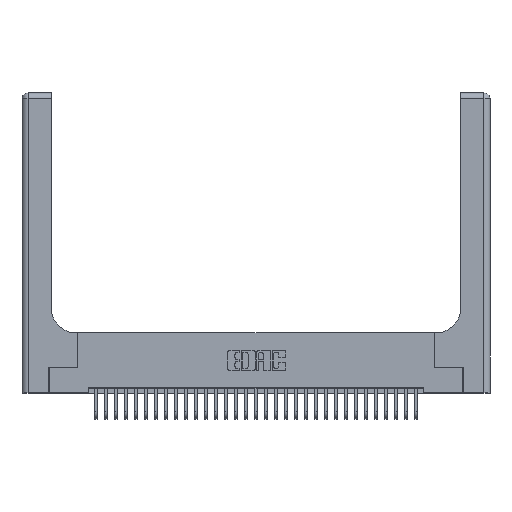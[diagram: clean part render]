
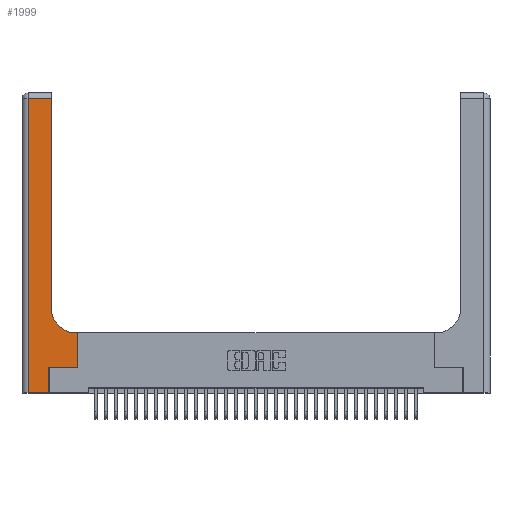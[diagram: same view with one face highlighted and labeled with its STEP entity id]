
A CAD part, top view. The second image highlights one B-rep face of the part: STEP entity #1999.
In plain terms, the highlighted planar face has unit normal (0, 0, 1).
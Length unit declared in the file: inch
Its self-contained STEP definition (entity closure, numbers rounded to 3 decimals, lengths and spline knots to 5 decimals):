
#424 = CARTESIAN_POINT ( 'NONE',  ( 0.5585, 0.25, 0.37 ) ) ;
#471 = VECTOR ( 'NONE', #10366, 39.37008 ) ;
#733 = VERTEX_POINT ( 'NONE', #4312 ) ;
#902 = CARTESIAN_POINT ( 'NONE',  ( 0.5585, 0.6, 0.37 ) ) ;
#1046 = EDGE_CURVE ( 'NONE', #733, #5427, #9000, .T. ) ;
#1478 = VERTEX_POINT ( 'NONE', #20765 ) ;
#1999 = ADVANCED_FACE ( 'NONE', ( #8933 ), #15204, .F. ) ;
#2007 = DIRECTION ( 'NONE',  ( 0., 0., -1. ) ) ;
#3588 = VECTOR ( 'NONE', #16304, 39.37008 ) ;
#3784 = EDGE_CURVE ( 'NONE', #26422, #733, #27342, .T. ) ;
#4034 = ORIENTED_EDGE ( 'NONE', *, *, #1046, .T. ) ;
#4134 = CARTESIAN_POINT ( 'NONE',  ( 0.2915, 0.6, 0.37 ) ) ;
#4312 = CARTESIAN_POINT ( 'NONE',  ( 0.5585, 0.25, 0.37 ) ) ;
#5159 = VECTOR ( 'NONE', #16176, 39.37008 ) ;
#5379 = CARTESIAN_POINT ( 'NONE',  ( 0.06, 0., 0.37 ) ) ;
#5427 = VERTEX_POINT ( 'NONE', #902 ) ;
#5568 = LINE ( 'NONE', #4134, #31736 ) ;
#5596 = VERTEX_POINT ( 'NONE', #30439 ) ;
#5608 = DIRECTION ( 'NONE',  ( 0., 1., 0. ) ) ;
#6018 = LINE ( 'NONE', #31418, #5159 ) ;
#6984 = ORIENTED_EDGE ( 'NONE', *, *, #32931, .T. ) ;
#7171 = CARTESIAN_POINT ( 'NONE',  ( 0.269, 0.25, 0.37 ) ) ;
#7640 = CARTESIAN_POINT ( 'NONE',  ( 0.5415, 0.85, 0.37 ) ) ;
#8471 = VECTOR ( 'NONE', #31565, 39.37008 ) ;
#8933 = FACE_OUTER_BOUND ( 'NONE', #31082, .T. ) ;
#9000 = LINE ( 'NONE', #424, #3588 ) ;
#10038 = CARTESIAN_POINT ( 'NONE',  ( 0.2915, 0.85, 0.37 ) ) ;
#10211 = VECTOR ( 'NONE', #29467, 39.37008 ) ;
#10279 = DIRECTION ( 'NONE',  ( 1., 0., 0. ) ) ;
#10366 = DIRECTION ( 'NONE',  ( 0., -1., 0. ) ) ;
#11176 = CARTESIAN_POINT ( 'NONE',  ( 0.269, 0., 0.37 ) ) ;
#12222 = AXIS2_PLACEMENT_3D ( 'NONE', #7640, #25995, #10279 ) ;
#12754 = ORIENTED_EDGE ( 'NONE', *, *, #29171, .T. ) ;
#13418 = VECTOR ( 'NONE', #23021, 39.37008 ) ;
#13706 = VERTEX_POINT ( 'NONE', #5379 ) ;
#13813 = CIRCLE ( 'NONE', #12222, 0.25 ) ;
#14595 = LINE ( 'NONE', #23476, #471 ) ;
#15184 = ORIENTED_EDGE ( 'NONE', *, *, #22018, .T. ) ;
#15204 = PLANE ( 'NONE',  #26793 ) ;
#15467 = LINE ( 'NONE', #15980, #8471 ) ;
#15773 = CARTESIAN_POINT ( 'NONE',  ( 0.269, 0.25, 0.37 ) ) ;
#15980 = CARTESIAN_POINT ( 'NONE',  ( 0., 2.94, 0.37 ) ) ;
#16176 = DIRECTION ( 'NONE',  ( 1., 0., 0. ) ) ;
#16304 = DIRECTION ( 'NONE',  ( 0., 1., 0. ) ) ;
#16443 = ORIENTED_EDGE ( 'NONE', *, *, #3784, .T. ) ;
#16960 = CARTESIAN_POINT ( 'NONE',  ( 0.5415, 0.6, 0.37 ) ) ;
#17666 = ORIENTED_EDGE ( 'NONE', *, *, #29625, .T. ) ;
#18730 = CARTESIAN_POINT ( 'NONE',  ( 0.2915, 3., 0.37 ) ) ;
#18929 = VERTEX_POINT ( 'NONE', #10038 ) ;
#20510 = DIRECTION ( 'NONE',  ( -1., 0., 0. ) ) ;
#20765 = CARTESIAN_POINT ( 'NONE',  ( 0.269, 0., 0.37 ) ) ;
#22018 = EDGE_CURVE ( 'NONE', #5596, #30344, #15467, .T. ) ;
#23021 = DIRECTION ( 'NONE',  ( 1., 0., 0. ) ) ;
#23476 = CARTESIAN_POINT ( 'NONE',  ( 0.06, 3., 0.37 ) ) ;
#23656 = CARTESIAN_POINT ( 'NONE',  ( 0.06, 2.94, 0.37 ) ) ;
#25995 = DIRECTION ( 'NONE',  ( 0., 0., -1. ) ) ;
#26170 = VECTOR ( 'NONE', #5608, 39.37008 ) ;
#26422 = VERTEX_POINT ( 'NONE', #15773 ) ;
#26793 = AXIS2_PLACEMENT_3D ( 'NONE', #33375, #2007, #20510 ) ;
#27342 = LINE ( 'NONE', #7171, #13418 ) ;
#27802 = DIRECTION ( 'NONE',  ( -1., 0., 0. ) ) ;
#28692 = EDGE_CURVE ( 'NONE', #13706, #1478, #6018, .T. ) ;
#28872 = VERTEX_POINT ( 'NONE', #16960 ) ;
#28984 = EDGE_CURVE ( 'NONE', #5427, #28872, #5568, .T. ) ;
#29171 = EDGE_CURVE ( 'NONE', #28872, #18929, #13813, .T. ) ;
#29467 = DIRECTION ( 'NONE',  ( 0., 1., 0. ) ) ;
#29625 = EDGE_CURVE ( 'NONE', #30344, #13706, #14595, .T. ) ;
#30254 = LINE ( 'NONE', #11176, #10211 ) ;
#30344 = VERTEX_POINT ( 'NONE', #23656 ) ;
#30439 = CARTESIAN_POINT ( 'NONE',  ( 0.2915, 2.94, 0.37 ) ) ;
#31082 = EDGE_LOOP ( 'NONE', ( #31861, #15184, #17666, #31485, #6984, #16443, #4034, #31896, #12754 ) ) ;
#31418 = CARTESIAN_POINT ( 'NONE',  ( 0., 0., 0.37 ) ) ;
#31485 = ORIENTED_EDGE ( 'NONE', *, *, #28692, .T. ) ;
#31565 = DIRECTION ( 'NONE',  ( -1., 0., 0. ) ) ;
#31736 = VECTOR ( 'NONE', #27802, 39.37008 ) ;
#31861 = ORIENTED_EDGE ( 'NONE', *, *, #33518, .T. ) ;
#31896 = ORIENTED_EDGE ( 'NONE', *, *, #28984, .T. ) ;
#32931 = EDGE_CURVE ( 'NONE', #1478, #26422, #30254, .T. ) ;
#33375 = CARTESIAN_POINT ( 'NONE',  ( 0., 3., 0.37 ) ) ;
#33518 = EDGE_CURVE ( 'NONE', #18929, #5596, #33800, .T. ) ;
#33800 = LINE ( 'NONE', #18730, #26170 ) ;
